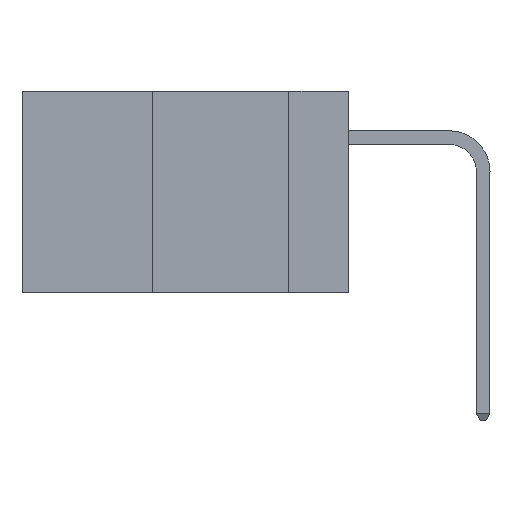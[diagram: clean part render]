
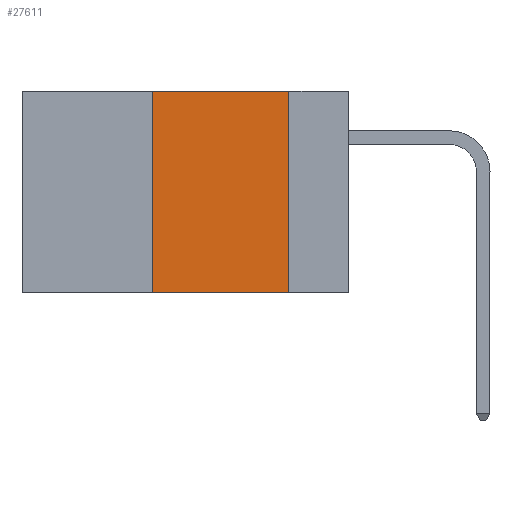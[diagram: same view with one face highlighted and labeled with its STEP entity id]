
A CAD part, left-side view. The second image highlights one B-rep face of the part: STEP entity #27611.
In plain terms, the highlighted planar face has unit normal (-1, 0, 0).
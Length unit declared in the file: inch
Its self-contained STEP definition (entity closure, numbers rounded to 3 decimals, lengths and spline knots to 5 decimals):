
#713 = CARTESIAN_POINT ( 'NONE',  ( 0., 0.6, -0.37 ) ) ;
#1136 = VERTEX_POINT ( 'NONE', #11208 ) ;
#1425 = CARTESIAN_POINT ( 'NONE',  ( 0., 0.36, 0. ) ) ;
#2023 = LINE ( 'NONE', #4789, #37872 ) ;
#3434 = DIRECTION ( 'NONE',  ( 0., -1., 0. ) ) ;
#3465 = VECTOR ( 'NONE', #10489, 39.37008 ) ;
#4520 = CARTESIAN_POINT ( 'NONE',  ( 0., 0.36, 0. ) ) ;
#4789 = CARTESIAN_POINT ( 'NONE',  ( 0., 0.11, 0. ) ) ;
#4821 = EDGE_CURVE ( 'NONE', #26074, #15909, #2023, .T. ) ;
#7746 = CARTESIAN_POINT ( 'NONE',  ( 0., 0.6, 0. ) ) ;
#7901 = EDGE_LOOP ( 'NONE', ( #29663, #8337, #12144, #37735 ) ) ;
#8337 = ORIENTED_EDGE ( 'NONE', *, *, #15130, .F. ) ;
#10489 = DIRECTION ( 'NONE',  ( 0., 0., 1. ) ) ;
#11208 = CARTESIAN_POINT ( 'NONE',  ( 0., 0.36, -0.37 ) ) ;
#12144 = ORIENTED_EDGE ( 'NONE', *, *, #15266, .F. ) ;
#13094 = VERTEX_POINT ( 'NONE', #1425 ) ;
#13227 = DIRECTION ( 'NONE',  ( 0., 0., -1. ) ) ;
#14299 = PLANE ( 'NONE',  #16183 ) ;
#15081 = LINE ( 'NONE', #4520, #3465 ) ;
#15130 = EDGE_CURVE ( 'NONE', #13094, #26074, #22552, .T. ) ;
#15266 = EDGE_CURVE ( 'NONE', #1136, #13094, #15081, .T. ) ;
#15909 = VERTEX_POINT ( 'NONE', #25672 ) ;
#16183 = AXIS2_PLACEMENT_3D ( 'NONE', #17308, #26404, #23386 ) ;
#17308 = CARTESIAN_POINT ( 'NONE',  ( 0., 0.6, 0. ) ) ;
#20263 = VECTOR ( 'NONE', #33135, 39.37008 ) ;
#22552 = LINE ( 'NONE', #7746, #23952 ) ;
#23386 = DIRECTION ( 'NONE',  ( 0., 0., -1. ) ) ;
#23952 = VECTOR ( 'NONE', #3434, 39.37008 ) ;
#25672 = CARTESIAN_POINT ( 'NONE',  ( 0., 0.11, -0.37 ) ) ;
#26051 = CARTESIAN_POINT ( 'NONE',  ( 0., 0.11, 0. ) ) ;
#26074 = VERTEX_POINT ( 'NONE', #26051 ) ;
#26404 = DIRECTION ( 'NONE',  ( 1., 0., 0. ) ) ;
#27611 = ADVANCED_FACE ( 'NONE', ( #38579 ), #14299, .F. ) ;
#29663 = ORIENTED_EDGE ( 'NONE', *, *, #4821, .F. ) ;
#33135 = DIRECTION ( 'NONE',  ( 0., -1., 0. ) ) ;
#36104 = LINE ( 'NONE', #713, #20263 ) ;
#37179 = EDGE_CURVE ( 'NONE', #1136, #15909, #36104, .T. ) ;
#37735 = ORIENTED_EDGE ( 'NONE', *, *, #37179, .T. ) ;
#37872 = VECTOR ( 'NONE', #13227, 39.37008 ) ;
#38579 = FACE_OUTER_BOUND ( 'NONE', #7901, .T. ) ;
